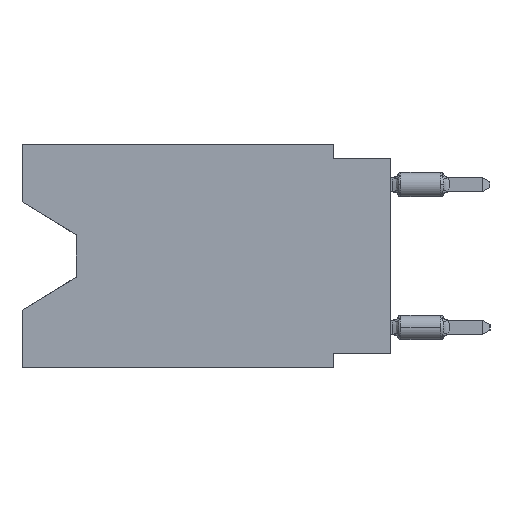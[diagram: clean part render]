
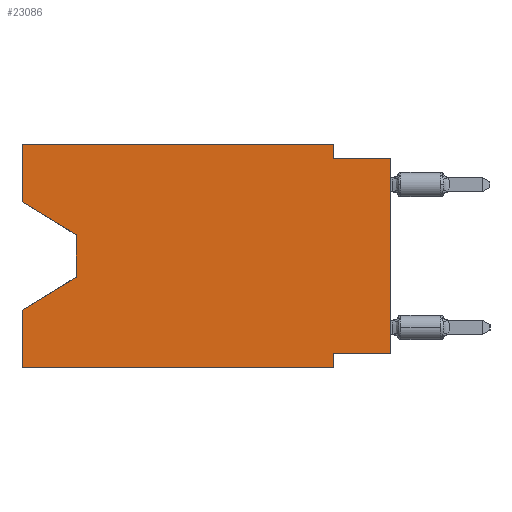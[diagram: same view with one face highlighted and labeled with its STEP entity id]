
A CAD part, left-side view. The second image highlights one B-rep face of the part: STEP entity #23086.
In plain terms, the highlighted planar face has unit normal (-1, 0, 0).
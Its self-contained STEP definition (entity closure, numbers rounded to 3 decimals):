
#95 = VECTOR ( 'NONE', #7477, 1000. ) ;
#379 = EDGE_CURVE ( 'NONE', #5726, #24089, #8434, .T. ) ;
#581 = CARTESIAN_POINT ( 'NONE',  ( 0., 16.383, -9.906 ) ) ;
#1059 = EDGE_CURVE ( 'NONE', #21684, #5726, #8199, .T. ) ;
#1099 = VECTOR ( 'NONE', #12149, 1000. ) ;
#1558 = LINE ( 'NONE', #17307, #18243 ) ;
#1821 = DIRECTION ( 'NONE',  ( 0., 0., 1. ) ) ;
#2267 = EDGE_CURVE ( 'NONE', #13787, #11947, #12027, .T. ) ;
#2358 = CARTESIAN_POINT ( 'NONE',  ( 0., 16.383, 0. ) ) ;
#2586 = VECTOR ( 'NONE', #8535, 1000. ) ;
#2836 = EDGE_CURVE ( 'NONE', #11129, #5335, #9214, .T. ) ;
#3121 = CARTESIAN_POINT ( 'NONE',  ( 0., 16.383, -2.546 ) ) ;
#3210 = CARTESIAN_POINT ( 'NONE',  ( 0., 16.383, -2.546 ) ) ;
#3577 = LINE ( 'NONE', #3210, #23363 ) ;
#3744 = CARTESIAN_POINT ( 'NONE',  ( 0., 0., -0.635 ) ) ;
#4179 = ORIENTED_EDGE ( 'NONE', *, *, #22603, .F. ) ;
#4215 = CARTESIAN_POINT ( 'NONE',  ( 0., 13.97, -4.013 ) ) ;
#4607 = CARTESIAN_POINT ( 'NONE',  ( 0., 16.383, 0. ) ) ;
#5335 = VERTEX_POINT ( 'NONE', #21972 ) ;
#5401 = CARTESIAN_POINT ( 'NONE',  ( 0., 2.54, 0. ) ) ;
#5726 = VERTEX_POINT ( 'NONE', #5933 ) ;
#5749 = VECTOR ( 'NONE', #22966, 1000. ) ;
#5933 = CARTESIAN_POINT ( 'NONE',  ( 0., 2.54, -9.271 ) ) ;
#6510 = EDGE_CURVE ( 'NONE', #21684, #5335, #25303, .T. ) ;
#6583 = CARTESIAN_POINT ( 'NONE',  ( 0., 2.54, -9.906 ) ) ;
#6733 = LINE ( 'NONE', #581, #2586 ) ;
#7290 = ORIENTED_EDGE ( 'NONE', *, *, #6510, .T. ) ;
#7477 = DIRECTION ( 'NONE',  ( 0., 0.855, -0.519 ) ) ;
#7705 = ORIENTED_EDGE ( 'NONE', *, *, #20865, .T. ) ;
#8059 = VERTEX_POINT ( 'NONE', #22243 ) ;
#8199 = LINE ( 'NONE', #21880, #21262 ) ;
#8246 = CARTESIAN_POINT ( 'NONE',  ( 0., 16.383, -9.906 ) ) ;
#8434 = LINE ( 'NONE', #24610, #15008 ) ;
#8535 = DIRECTION ( 'NONE',  ( 0., -1., 0. ) ) ;
#9064 = EDGE_CURVE ( 'NONE', #12115, #20924, #10577, .T. ) ;
#9158 = DIRECTION ( 'NONE',  ( 0., 0., -1. ) ) ;
#9214 = LINE ( 'NONE', #3744, #25676 ) ;
#9902 = DIRECTION ( 'NONE',  ( 0., 1., 0. ) ) ;
#9988 = ORIENTED_EDGE ( 'NONE', *, *, #1059, .F. ) ;
#10519 = EDGE_LOOP ( 'NONE', ( #19815, #13791, #12218, #13525, #7705, #22784, #9988, #7290, #22420, #4179, #12895, #14715 ) ) ;
#10577 = LINE ( 'NONE', #4607, #5749 ) ;
#11102 = LINE ( 'NONE', #5401, #25394 ) ;
#11129 = VERTEX_POINT ( 'NONE', #23963 ) ;
#11458 = DIRECTION ( 'NONE',  ( 0., 0., -1. ) ) ;
#11947 = VERTEX_POINT ( 'NONE', #13816 ) ;
#12027 = LINE ( 'NONE', #4215, #1099 ) ;
#12115 = VERTEX_POINT ( 'NONE', #3121 ) ;
#12149 = DIRECTION ( 'NONE',  ( 0., 0., -1. ) ) ;
#12218 = ORIENTED_EDGE ( 'NONE', *, *, #18637, .T. ) ;
#12244 = VERTEX_POINT ( 'NONE', #20852 ) ;
#12895 = ORIENTED_EDGE ( 'NONE', *, *, #21775, .F. ) ;
#13339 = CARTESIAN_POINT ( 'NONE',  ( 0., 13.97, -5.893 ) ) ;
#13525 = ORIENTED_EDGE ( 'NONE', *, *, #16534, .F. ) ;
#13782 = VECTOR ( 'NONE', #18635, 1000. ) ;
#13787 = VERTEX_POINT ( 'NONE', #15240 ) ;
#13791 = ORIENTED_EDGE ( 'NONE', *, *, #2267, .T. ) ;
#13816 = CARTESIAN_POINT ( 'NONE',  ( 0., 13.97, -5.893 ) ) ;
#14715 = ORIENTED_EDGE ( 'NONE', *, *, #9064, .F. ) ;
#15008 = VECTOR ( 'NONE', #24342, 1000. ) ;
#15240 = CARTESIAN_POINT ( 'NONE',  ( 0., 13.97, -4.013 ) ) ;
#16534 = EDGE_CURVE ( 'NONE', #21217, #8059, #24391, .T. ) ;
#17052 = EDGE_CURVE ( 'NONE', #12115, #13787, #3577, .T. ) ;
#17154 = DIRECTION ( 'NONE',  ( 0., -1., 0. ) ) ;
#17307 = CARTESIAN_POINT ( 'NONE',  ( 0., 16.383, 0. ) ) ;
#17359 = LINE ( 'NONE', #13339, #95 ) ;
#17831 = PLANE ( 'NONE',  #24882 ) ;
#18243 = VECTOR ( 'NONE', #25173, 1000. ) ;
#18635 = DIRECTION ( 'NONE',  ( 0., 0., 1. ) ) ;
#18637 = EDGE_CURVE ( 'NONE', #11947, #8059, #17359, .T. ) ;
#19204 = VECTOR ( 'NONE', #1821, 1000. ) ;
#19482 = DIRECTION ( 'NONE',  ( 0., -0.855, -0.519 ) ) ;
#19674 = CARTESIAN_POINT ( 'NONE',  ( 0., 0., 0. ) ) ;
#19815 = ORIENTED_EDGE ( 'NONE', *, *, #17052, .T. ) ;
#20852 = CARTESIAN_POINT ( 'NONE',  ( 0., 2.54, 0. ) ) ;
#20865 = EDGE_CURVE ( 'NONE', #21217, #24089, #6733, .T. ) ;
#20924 = VERTEX_POINT ( 'NONE', #20930 ) ;
#20930 = CARTESIAN_POINT ( 'NONE',  ( 0., 16.383, 0. ) ) ;
#21217 = VERTEX_POINT ( 'NONE', #8246 ) ;
#21250 = DIRECTION ( 'NONE',  ( 1., 0., 0. ) ) ;
#21262 = VECTOR ( 'NONE', #9902, 1000. ) ;
#21375 = FACE_OUTER_BOUND ( 'NONE', #10519, .T. ) ;
#21684 = VERTEX_POINT ( 'NONE', #24921 ) ;
#21775 = EDGE_CURVE ( 'NONE', #20924, #12244, #1558, .T. ) ;
#21880 = CARTESIAN_POINT ( 'NONE',  ( 0., 0., -9.271 ) ) ;
#21972 = CARTESIAN_POINT ( 'NONE',  ( 0., 0., -0.635 ) ) ;
#22243 = CARTESIAN_POINT ( 'NONE',  ( 0., 16.383, -7.36 ) ) ;
#22420 = ORIENTED_EDGE ( 'NONE', *, *, #2836, .F. ) ;
#22603 = EDGE_CURVE ( 'NONE', #12244, #11129, #11102, .T. ) ;
#22784 = ORIENTED_EDGE ( 'NONE', *, *, #379, .F. ) ;
#22966 = DIRECTION ( 'NONE',  ( 0., 0., 1. ) ) ;
#23086 = ADVANCED_FACE ( 'NONE', ( #21375 ), #17831, .F. ) ;
#23363 = VECTOR ( 'NONE', #19482, 1000. ) ;
#23845 = CARTESIAN_POINT ( 'NONE',  ( 0., 16.383, 0. ) ) ;
#23963 = CARTESIAN_POINT ( 'NONE',  ( 0., 2.54, -0.635 ) ) ;
#24089 = VERTEX_POINT ( 'NONE', #6583 ) ;
#24342 = DIRECTION ( 'NONE',  ( 0., 0., -1. ) ) ;
#24391 = LINE ( 'NONE', #2358, #13782 ) ;
#24610 = CARTESIAN_POINT ( 'NONE',  ( 0., 2.54, -9.906 ) ) ;
#24882 = AXIS2_PLACEMENT_3D ( 'NONE', #23845, #21250, #11458 ) ;
#24921 = CARTESIAN_POINT ( 'NONE',  ( 0., 0., -9.271 ) ) ;
#25173 = DIRECTION ( 'NONE',  ( 0., -1., 0. ) ) ;
#25303 = LINE ( 'NONE', #19674, #19204 ) ;
#25394 = VECTOR ( 'NONE', #9158, 1000. ) ;
#25676 = VECTOR ( 'NONE', #17154, 1000. ) ;
